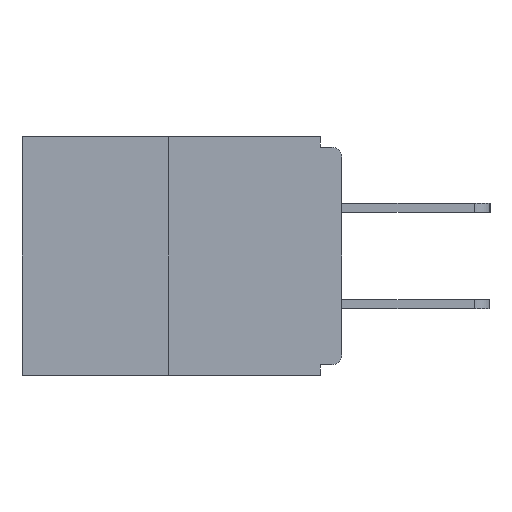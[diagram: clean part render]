
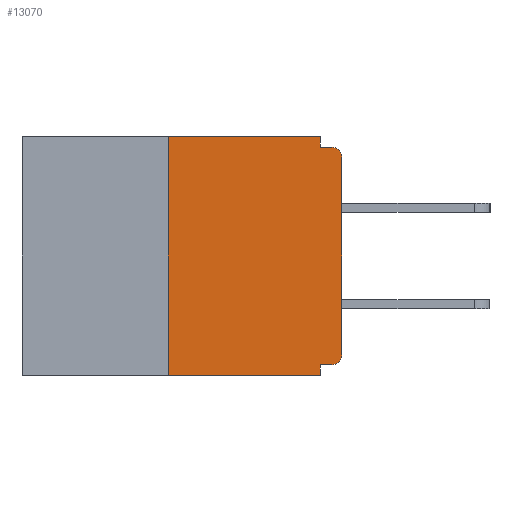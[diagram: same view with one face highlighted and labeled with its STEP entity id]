
A CAD part, left-side view. The second image highlights one B-rep face of the part: STEP entity #13070.
In plain terms, the highlighted planar face has unit normal (-1, 0, 0).
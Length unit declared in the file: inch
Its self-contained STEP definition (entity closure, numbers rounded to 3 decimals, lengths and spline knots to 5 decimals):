
#75 = DIRECTION ( 'NONE',  ( -1., 0., 0. ) ) ;
#501 = ORIENTED_EDGE ( 'NONE', *, *, #1487, .F. ) ;
#670 = EDGE_CURVE ( 'NONE', #3268, #14457, #10291, .T. ) ;
#685 = VECTOR ( 'NONE', #6087, 39.37008 ) ;
#731 = VECTOR ( 'NONE', #8498, 39.37008 ) ;
#1304 = DIRECTION ( 'NONE',  ( 0., 0., -1. ) ) ;
#1314 = EDGE_CURVE ( 'NONE', #5386, #11292, #11418, .T. ) ;
#1378 = ORIENTED_EDGE ( 'NONE', *, *, #670, .F. ) ;
#1440 = VERTEX_POINT ( 'NONE', #4721 ) ;
#1487 = EDGE_CURVE ( 'NONE', #14457, #12827, #4571, .T. ) ;
#1492 = EDGE_CURVE ( 'NONE', #11292, #10339, #1606, .T. ) ;
#1518 = EDGE_LOOP ( 'NONE', ( #501, #1378, #7762, #13830, #4521, #14144, #4146, #7643, #11607, #15293 ) ) ;
#1606 = LINE ( 'NONE', #3465, #685 ) ;
#1873 = CIRCLE ( 'NONE', #13823, 0.015 ) ;
#1886 = CARTESIAN_POINT ( 'NONE',  ( 0., 0.015, -0.313 ) ) ;
#2206 = CARTESIAN_POINT ( 'NONE',  ( 0., 0., -0.015 ) ) ;
#2298 = LINE ( 'NONE', #5950, #14764 ) ;
#2453 = PLANE ( 'NONE',  #13431 ) ;
#2472 = CARTESIAN_POINT ( 'NONE',  ( 0., 0.031, -0.343 ) ) ;
#2528 = DIRECTION ( 'NONE',  ( 0., 0., 1. ) ) ;
#2987 = CARTESIAN_POINT ( 'NONE',  ( 0., 0.25, -0.343 ) ) ;
#3268 = VERTEX_POINT ( 'NONE', #2987 ) ;
#3465 = CARTESIAN_POINT ( 'NONE',  ( 0., 0.031, -0.343 ) ) ;
#3487 = DIRECTION ( 'NONE',  ( 0., -1., 0. ) ) ;
#3566 = LINE ( 'NONE', #15577, #13399 ) ;
#3839 = CARTESIAN_POINT ( 'NONE',  ( 0., 0.015, -0.03 ) ) ;
#3878 = VECTOR ( 'NONE', #11092, 39.37008 ) ;
#4146 = ORIENTED_EDGE ( 'NONE', *, *, #11934, .T. ) ;
#4521 = ORIENTED_EDGE ( 'NONE', *, *, #1314, .F. ) ;
#4571 = LINE ( 'NONE', #4864, #12556 ) ;
#4721 = CARTESIAN_POINT ( 'NONE',  ( 0., 0.015, -0.015 ) ) ;
#4776 = EDGE_CURVE ( 'NONE', #3268, #10339, #3566, .T. ) ;
#4804 = EDGE_CURVE ( 'NONE', #5386, #10904, #1873, .T. ) ;
#4837 = DIRECTION ( 'NONE',  ( 1., 0., 0. ) ) ;
#4864 = CARTESIAN_POINT ( 'NONE',  ( 0., 0.46, 0. ) ) ;
#5214 = CARTESIAN_POINT ( 'NONE',  ( 0., 0.015, -0.328 ) ) ;
#5250 = CIRCLE ( 'NONE', #7864, 0.015 ) ;
#5386 = VERTEX_POINT ( 'NONE', #5214 ) ;
#5768 = CARTESIAN_POINT ( 'NONE',  ( 0., 0.031, -0.328 ) ) ;
#5950 = CARTESIAN_POINT ( 'NONE',  ( 0., 0.031, 0. ) ) ;
#6087 = DIRECTION ( 'NONE',  ( 0., 0., -1. ) ) ;
#6699 = EDGE_CURVE ( 'NONE', #12203, #1440, #10129, .T. ) ;
#7417 = CARTESIAN_POINT ( 'NONE',  ( 0., 0., 0. ) ) ;
#7601 = FACE_OUTER_BOUND ( 'NONE', #1518, .T. ) ;
#7643 = ORIENTED_EDGE ( 'NONE', *, *, #14309, .T. ) ;
#7762 = ORIENTED_EDGE ( 'NONE', *, *, #4776, .T. ) ;
#7864 = AXIS2_PLACEMENT_3D ( 'NONE', #3839, #75, #12306 ) ;
#8197 = VECTOR ( 'NONE', #10034, 39.37008 ) ;
#8446 = VERTEX_POINT ( 'NONE', #10951 ) ;
#8498 = DIRECTION ( 'NONE',  ( 0., -1., 0. ) ) ;
#8690 = DIRECTION ( 'NONE',  ( 0., 0., -1. ) ) ;
#8820 = CARTESIAN_POINT ( 'NONE',  ( 0., 0.25, 0. ) ) ;
#9085 = CARTESIAN_POINT ( 'NONE',  ( 0., 0., -0.313 ) ) ;
#9497 = CARTESIAN_POINT ( 'NONE',  ( 0., 0.031, -0.015 ) ) ;
#9626 = DIRECTION ( 'NONE',  ( 0., -1., 0. ) ) ;
#10034 = DIRECTION ( 'NONE',  ( 0., 1., 0. ) ) ;
#10129 = LINE ( 'NONE', #2206, #731 ) ;
#10291 = LINE ( 'NONE', #8820, #3878 ) ;
#10339 = VERTEX_POINT ( 'NONE', #2472 ) ;
#10363 = DIRECTION ( 'NONE',  ( -1., 0., 0. ) ) ;
#10572 = CARTESIAN_POINT ( 'NONE',  ( 0., 0.25, 0. ) ) ;
#10904 = VERTEX_POINT ( 'NONE', #9085 ) ;
#10951 = CARTESIAN_POINT ( 'NONE',  ( 0., 0., -0.03 ) ) ;
#11092 = DIRECTION ( 'NONE',  ( 0., 0., 1. ) ) ;
#11292 = VERTEX_POINT ( 'NONE', #5768 ) ;
#11418 = LINE ( 'NONE', #14687, #8197 ) ;
#11607 = ORIENTED_EDGE ( 'NONE', *, *, #6699, .F. ) ;
#11934 = EDGE_CURVE ( 'NONE', #10904, #8446, #12372, .T. ) ;
#12118 = CARTESIAN_POINT ( 'NONE',  ( 0., 0.46, 0. ) ) ;
#12203 = VERTEX_POINT ( 'NONE', #9497 ) ;
#12306 = DIRECTION ( 'NONE',  ( 0., 0., -1. ) ) ;
#12372 = LINE ( 'NONE', #7417, #12738 ) ;
#12556 = VECTOR ( 'NONE', #9626, 39.37008 ) ;
#12738 = VECTOR ( 'NONE', #2528, 39.37008 ) ;
#12827 = VERTEX_POINT ( 'NONE', #14702 ) ;
#13070 = ADVANCED_FACE ( 'NONE', ( #7601 ), #2453, .F. ) ;
#13192 = EDGE_CURVE ( 'NONE', #12827, #12203, #2298, .T. ) ;
#13399 = VECTOR ( 'NONE', #3487, 39.37008 ) ;
#13431 = AXIS2_PLACEMENT_3D ( 'NONE', #12118, #4837, #1304 ) ;
#13823 = AXIS2_PLACEMENT_3D ( 'NONE', #1886, #10363, #14078 ) ;
#13830 = ORIENTED_EDGE ( 'NONE', *, *, #1492, .F. ) ;
#14078 = DIRECTION ( 'NONE',  ( 0., 0., -1. ) ) ;
#14144 = ORIENTED_EDGE ( 'NONE', *, *, #4804, .T. ) ;
#14309 = EDGE_CURVE ( 'NONE', #8446, #1440, #5250, .T. ) ;
#14457 = VERTEX_POINT ( 'NONE', #10572 ) ;
#14687 = CARTESIAN_POINT ( 'NONE',  ( 0., 0., -0.328 ) ) ;
#14702 = CARTESIAN_POINT ( 'NONE',  ( 0., 0.031, 0. ) ) ;
#14764 = VECTOR ( 'NONE', #8690, 39.37008 ) ;
#15293 = ORIENTED_EDGE ( 'NONE', *, *, #13192, .F. ) ;
#15577 = CARTESIAN_POINT ( 'NONE',  ( 0., 0.46, -0.343 ) ) ;
